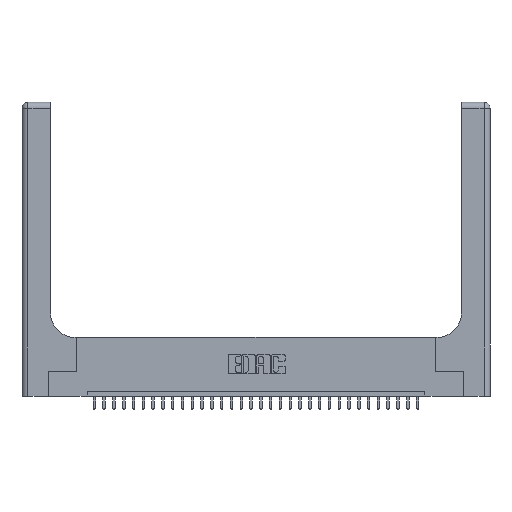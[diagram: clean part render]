
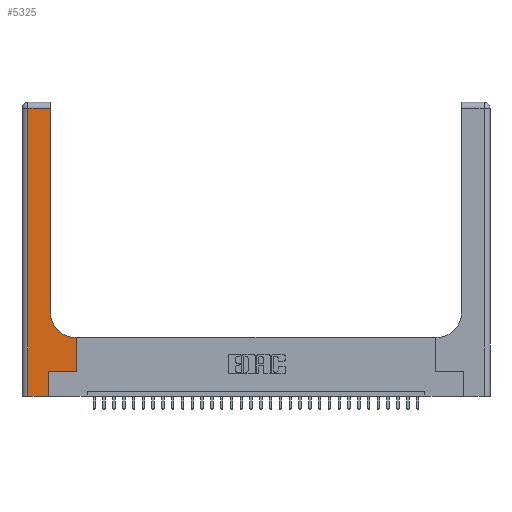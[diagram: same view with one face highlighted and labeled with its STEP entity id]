
A CAD part, top view. The second image highlights one B-rep face of the part: STEP entity #5325.
In plain terms, the highlighted planar face has unit normal (0, 0, 1).
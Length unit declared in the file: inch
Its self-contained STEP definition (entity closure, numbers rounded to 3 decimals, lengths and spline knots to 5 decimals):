
#825 = EDGE_CURVE ( 'NONE', #24643, #15217, #1036, .T. ) ;
#909 = CARTESIAN_POINT ( 'NONE',  ( 0.5585, 0.25, 0.37 ) ) ;
#967 = CARTESIAN_POINT ( 'NONE',  ( 0.06, 0., 0.37 ) ) ;
#1036 = LINE ( 'NONE', #29000, #26472 ) ;
#1710 = LINE ( 'NONE', #18438, #15966 ) ;
#2265 = ORIENTED_EDGE ( 'NONE', *, *, #9316, .T. ) ;
#2685 = VERTEX_POINT ( 'NONE', #27538 ) ;
#3634 = AXIS2_PLACEMENT_3D ( 'NONE', #16048, #28647, #27998 ) ;
#3907 = VERTEX_POINT ( 'NONE', #23757 ) ;
#4601 = CIRCLE ( 'NONE', #25428, 0.25 ) ;
#5157 = DIRECTION ( 'NONE',  ( 1., 0., 0. ) ) ;
#5325 = ADVANCED_FACE ( 'NONE', ( #22941 ), #26452, .F. ) ;
#5646 = EDGE_LOOP ( 'NONE', ( #15481, #23199, #24666, #15605, #26105, #16250, #6096, #2265, #6509 ) ) ;
#6096 = ORIENTED_EDGE ( 'NONE', *, *, #20039, .T. ) ;
#6455 = CARTESIAN_POINT ( 'NONE',  ( 0.5585, 0.25, 0.37 ) ) ;
#6509 = ORIENTED_EDGE ( 'NONE', *, *, #26148, .T. ) ;
#6875 = EDGE_CURVE ( 'NONE', #14329, #14646, #7802, .T. ) ;
#7802 = LINE ( 'NONE', #27181, #30533 ) ;
#8384 = VECTOR ( 'NONE', #28253, 39.37008 ) ;
#8613 = EDGE_CURVE ( 'NONE', #2685, #16640, #20425, .T. ) ;
#9316 = EDGE_CURVE ( 'NONE', #20055, #12158, #14936, .T. ) ;
#11714 = LINE ( 'NONE', #28855, #15954 ) ;
#12158 = VERTEX_POINT ( 'NONE', #22992 ) ;
#13254 = CARTESIAN_POINT ( 'NONE',  ( 0.269, 0., 0.37 ) ) ;
#13627 = CARTESIAN_POINT ( 'NONE',  ( 0.269, 0.25, 0.37 ) ) ;
#13885 = DIRECTION ( 'NONE',  ( 0., 1., 0. ) ) ;
#14329 = VERTEX_POINT ( 'NONE', #29121 ) ;
#14646 = VERTEX_POINT ( 'NONE', #967 ) ;
#14936 = LINE ( 'NONE', #16725, #8384 ) ;
#15217 = VERTEX_POINT ( 'NONE', #909 ) ;
#15481 = ORIENTED_EDGE ( 'NONE', *, *, #8613, .T. ) ;
#15605 = ORIENTED_EDGE ( 'NONE', *, *, #28574, .T. ) ;
#15954 = VECTOR ( 'NONE', #30979, 39.37008 ) ;
#15966 = VECTOR ( 'NONE', #26003, 39.37008 ) ;
#16048 = CARTESIAN_POINT ( 'NONE',  ( 0., 3., 0.37 ) ) ;
#16250 = ORIENTED_EDGE ( 'NONE', *, *, #825, .T. ) ;
#16405 = DIRECTION ( 'NONE',  ( 1., 0., 0. ) ) ;
#16640 = VERTEX_POINT ( 'NONE', #26505 ) ;
#16725 = CARTESIAN_POINT ( 'NONE',  ( 0.2915, 0.6, 0.37 ) ) ;
#16817 = VECTOR ( 'NONE', #30469, 39.37008 ) ;
#18201 = LINE ( 'NONE', #6455, #21315 ) ;
#18438 = CARTESIAN_POINT ( 'NONE',  ( 0., 2.94, 0.37 ) ) ;
#19414 = EDGE_CURVE ( 'NONE', #16640, #14329, #1710, .T. ) ;
#19834 = DIRECTION ( 'NONE',  ( 0., -1., 0. ) ) ;
#20039 = EDGE_CURVE ( 'NONE', #15217, #20055, #18201, .T. ) ;
#20055 = VERTEX_POINT ( 'NONE', #30787 ) ;
#20425 = LINE ( 'NONE', #28349, #29310 ) ;
#21315 = VECTOR ( 'NONE', #13885, 39.37008 ) ;
#22191 = CARTESIAN_POINT ( 'NONE',  ( 0.5415, 0.85, 0.37 ) ) ;
#22941 = FACE_OUTER_BOUND ( 'NONE', #5646, .T. ) ;
#22992 = CARTESIAN_POINT ( 'NONE',  ( 0.5415, 0.6, 0.37 ) ) ;
#23199 = ORIENTED_EDGE ( 'NONE', *, *, #19414, .T. ) ;
#23757 = CARTESIAN_POINT ( 'NONE',  ( 0.269, 0., 0.37 ) ) ;
#23779 = LINE ( 'NONE', #13254, #16817 ) ;
#24643 = VERTEX_POINT ( 'NONE', #13627 ) ;
#24666 = ORIENTED_EDGE ( 'NONE', *, *, #6875, .T. ) ;
#25428 = AXIS2_PLACEMENT_3D ( 'NONE', #22191, #27351, #5157 ) ;
#25798 = DIRECTION ( 'NONE',  ( 0., 1., 0. ) ) ;
#26003 = DIRECTION ( 'NONE',  ( -1., 0., 0. ) ) ;
#26105 = ORIENTED_EDGE ( 'NONE', *, *, #27411, .T. ) ;
#26148 = EDGE_CURVE ( 'NONE', #12158, #2685, #4601, .T. ) ;
#26452 = PLANE ( 'NONE',  #3634 ) ;
#26472 = VECTOR ( 'NONE', #16405, 39.37008 ) ;
#26505 = CARTESIAN_POINT ( 'NONE',  ( 0.2915, 2.94, 0.37 ) ) ;
#27181 = CARTESIAN_POINT ( 'NONE',  ( 0.06, 3., 0.37 ) ) ;
#27351 = DIRECTION ( 'NONE',  ( 0., 0., -1. ) ) ;
#27411 = EDGE_CURVE ( 'NONE', #3907, #24643, #23779, .T. ) ;
#27538 = CARTESIAN_POINT ( 'NONE',  ( 0.2915, 0.85, 0.37 ) ) ;
#27998 = DIRECTION ( 'NONE',  ( -1., 0., 0. ) ) ;
#28253 = DIRECTION ( 'NONE',  ( -1., 0., 0. ) ) ;
#28349 = CARTESIAN_POINT ( 'NONE',  ( 0.2915, 3., 0.37 ) ) ;
#28574 = EDGE_CURVE ( 'NONE', #14646, #3907, #11714, .T. ) ;
#28647 = DIRECTION ( 'NONE',  ( 0., 0., -1. ) ) ;
#28855 = CARTESIAN_POINT ( 'NONE',  ( 0., 0., 0.37 ) ) ;
#29000 = CARTESIAN_POINT ( 'NONE',  ( 0.269, 0.25, 0.37 ) ) ;
#29121 = CARTESIAN_POINT ( 'NONE',  ( 0.06, 2.94, 0.37 ) ) ;
#29310 = VECTOR ( 'NONE', #25798, 39.37008 ) ;
#30469 = DIRECTION ( 'NONE',  ( 0., 1., 0. ) ) ;
#30533 = VECTOR ( 'NONE', #19834, 39.37008 ) ;
#30787 = CARTESIAN_POINT ( 'NONE',  ( 0.5585, 0.6, 0.37 ) ) ;
#30979 = DIRECTION ( 'NONE',  ( 1., 0., 0. ) ) ;
